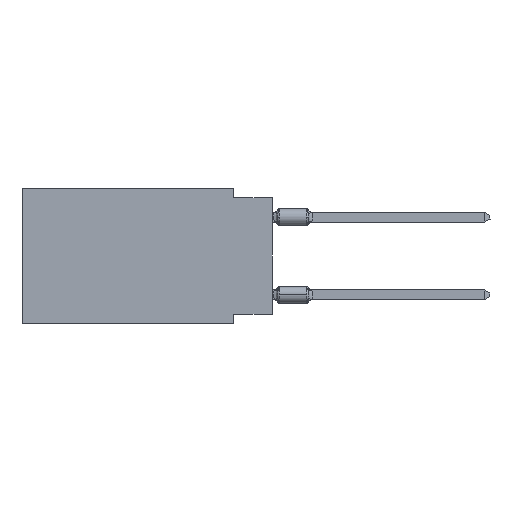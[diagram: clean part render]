
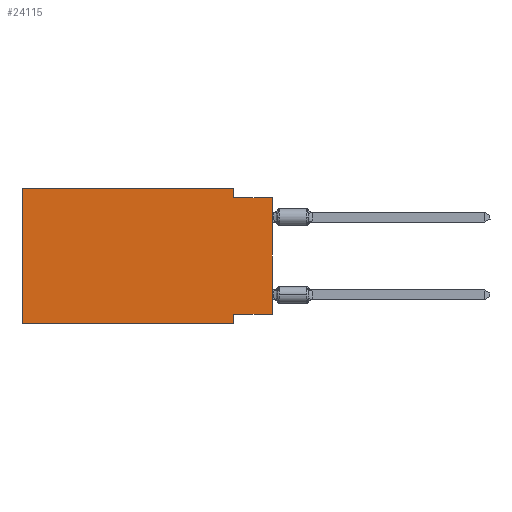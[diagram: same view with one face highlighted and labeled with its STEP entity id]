
A CAD part, left-side view. The second image highlights one B-rep face of the part: STEP entity #24115.
In plain terms, the highlighted planar face has unit normal (-1, 0, 0).
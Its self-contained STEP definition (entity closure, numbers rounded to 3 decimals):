
#22 = CARTESIAN_POINT ( 'NONE',  ( 0., 2.54, -8.255 ) ) ;
#583 = VECTOR ( 'NONE', #60905, 1000. ) ;
#931 = CARTESIAN_POINT ( 'NONE',  ( 0., 0., -0.635 ) ) ;
#1072 = VECTOR ( 'NONE', #15551, 1000. ) ;
#1555 = LINE ( 'NONE', #6513, #1072 ) ;
#3759 = CARTESIAN_POINT ( 'NONE',  ( 0., 16.383, -8.89 ) ) ;
#4373 = VECTOR ( 'NONE', #29946, 1000. ) ;
#5101 = CARTESIAN_POINT ( 'NONE',  ( 0., 16.383, 0. ) ) ;
#6513 = CARTESIAN_POINT ( 'NONE',  ( 0., 0., -0.635 ) ) ;
#6523 = DIRECTION ( 'NONE',  ( 0., -1., 0. ) ) ;
#7652 = ORIENTED_EDGE ( 'NONE', *, *, #34164, .T. ) ;
#7709 = CARTESIAN_POINT ( 'NONE',  ( 0., 16.383, 0. ) ) ;
#7825 = EDGE_CURVE ( 'NONE', #21101, #26748, #40914, .T. ) ;
#8356 = CARTESIAN_POINT ( 'NONE',  ( 0., 2.54, -0.635 ) ) ;
#11054 = VERTEX_POINT ( 'NONE', #931 ) ;
#11879 = AXIS2_PLACEMENT_3D ( 'NONE', #5101, #13521, #43318 ) ;
#12055 = VECTOR ( 'NONE', #59865, 1000. ) ;
#12069 = ORIENTED_EDGE ( 'NONE', *, *, #60250, .F. ) ;
#13106 = ORIENTED_EDGE ( 'NONE', *, *, #30690, .F. ) ;
#13521 = DIRECTION ( 'NONE',  ( 1., 0., 0. ) ) ;
#14126 = FACE_OUTER_BOUND ( 'NONE', #43013, .T. ) ;
#15551 = DIRECTION ( 'NONE',  ( 0., -1., 0. ) ) ;
#16991 = EDGE_CURVE ( 'NONE', #34999, #48436, #20299, .T. ) ;
#18412 = ORIENTED_EDGE ( 'NONE', *, *, #46802, .F. ) ;
#19078 = EDGE_CURVE ( 'NONE', #34999, #11054, #23009, .T. ) ;
#20299 = LINE ( 'NONE', #26193, #34131 ) ;
#20848 = LINE ( 'NONE', #53141, #46266 ) ;
#21101 = VERTEX_POINT ( 'NONE', #25732 ) ;
#22991 = LINE ( 'NONE', #55602, #28235 ) ;
#23009 = LINE ( 'NONE', #41935, #583 ) ;
#23468 = PLANE ( 'NONE',  #11879 ) ;
#23603 = CARTESIAN_POINT ( 'NONE',  ( 0., 16.383, 0. ) ) ;
#23718 = ORIENTED_EDGE ( 'NONE', *, *, #7825, .F. ) ;
#24115 = ADVANCED_FACE ( 'NONE', ( #14126 ), #23468, .F. ) ;
#25615 = ORIENTED_EDGE ( 'NONE', *, *, #32378, .F. ) ;
#25732 = CARTESIAN_POINT ( 'NONE',  ( 0., 2.54, 0. ) ) ;
#25887 = DIRECTION ( 'NONE',  ( 0., 1., 0. ) ) ;
#26193 = CARTESIAN_POINT ( 'NONE',  ( 0., 0., -8.255 ) ) ;
#26748 = VERTEX_POINT ( 'NONE', #8356 ) ;
#26999 = DIRECTION ( 'NONE',  ( 0., -1., 0. ) ) ;
#28235 = VECTOR ( 'NONE', #46295, 1000. ) ;
#28794 = CARTESIAN_POINT ( 'NONE',  ( 0., 0., -8.255 ) ) ;
#29946 = DIRECTION ( 'NONE',  ( 0., 0., -1. ) ) ;
#30690 = EDGE_CURVE ( 'NONE', #39194, #55458, #22991, .T. ) ;
#30995 = CARTESIAN_POINT ( 'NONE',  ( 0., 2.54, 0. ) ) ;
#31197 = VECTOR ( 'NONE', #26999, 1000. ) ;
#32378 = EDGE_CURVE ( 'NONE', #55458, #21101, #50602, .T. ) ;
#34131 = VECTOR ( 'NONE', #25887, 1000. ) ;
#34164 = EDGE_CURVE ( 'NONE', #39194, #49537, #20848, .T. ) ;
#34902 = LINE ( 'NONE', #38947, #4373 ) ;
#34999 = VERTEX_POINT ( 'NONE', #28794 ) ;
#38323 = ORIENTED_EDGE ( 'NONE', *, *, #19078, .T. ) ;
#38947 = CARTESIAN_POINT ( 'NONE',  ( 0., 2.54, -8.89 ) ) ;
#39194 = VERTEX_POINT ( 'NONE', #3759 ) ;
#40914 = LINE ( 'NONE', #30995, #12055 ) ;
#41935 = CARTESIAN_POINT ( 'NONE',  ( 0., 0., 0. ) ) ;
#43013 = EDGE_LOOP ( 'NONE', ( #38323, #18412, #23718, #25615, #13106, #7652, #12069, #52177 ) ) ;
#43318 = DIRECTION ( 'NONE',  ( 0., 0., -1. ) ) ;
#46266 = VECTOR ( 'NONE', #6523, 1000. ) ;
#46295 = DIRECTION ( 'NONE',  ( 0., 0., 1. ) ) ;
#46802 = EDGE_CURVE ( 'NONE', #26748, #11054, #1555, .T. ) ;
#48436 = VERTEX_POINT ( 'NONE', #22 ) ;
#49537 = VERTEX_POINT ( 'NONE', #52397 ) ;
#50602 = LINE ( 'NONE', #7709, #31197 ) ;
#52177 = ORIENTED_EDGE ( 'NONE', *, *, #16991, .F. ) ;
#52397 = CARTESIAN_POINT ( 'NONE',  ( 0., 2.54, -8.89 ) ) ;
#53141 = CARTESIAN_POINT ( 'NONE',  ( 0., 16.383, -8.89 ) ) ;
#55458 = VERTEX_POINT ( 'NONE', #23603 ) ;
#55602 = CARTESIAN_POINT ( 'NONE',  ( 0., 16.383, 0. ) ) ;
#59865 = DIRECTION ( 'NONE',  ( 0., 0., -1. ) ) ;
#60250 = EDGE_CURVE ( 'NONE', #48436, #49537, #34902, .T. ) ;
#60905 = DIRECTION ( 'NONE',  ( 0., 0., 1. ) ) ;
